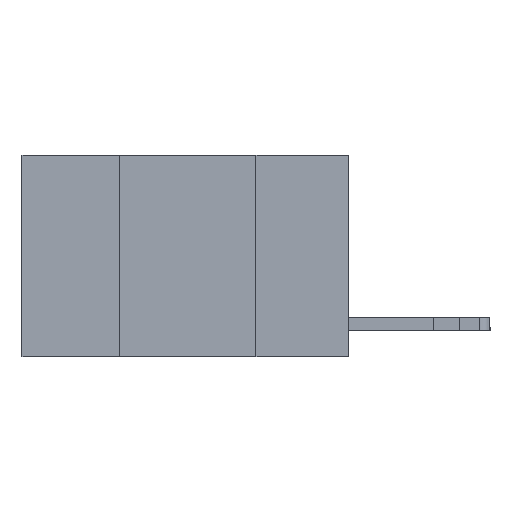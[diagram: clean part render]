
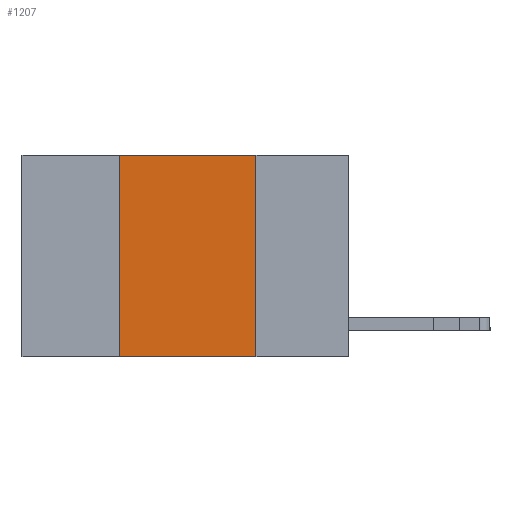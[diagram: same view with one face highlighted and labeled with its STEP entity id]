
A CAD part, left-side view. The second image highlights one B-rep face of the part: STEP entity #1207.
In plain terms, the highlighted planar face has unit normal (-1, 0, 0).
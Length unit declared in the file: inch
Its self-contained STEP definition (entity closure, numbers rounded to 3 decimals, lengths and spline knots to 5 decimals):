
#276 = ORIENTED_EDGE ( 'NONE', *, *, #12106, .F. ) ;
#777 = CARTESIAN_POINT ( 'NONE',  ( 0., 0.17, 0. ) ) ;
#1207 = ADVANCED_FACE ( 'NONE', ( #3936 ), #2541, .F. ) ;
#1278 = AXIS2_PLACEMENT_3D ( 'NONE', #9747, #12236, #2841 ) ;
#1428 = CARTESIAN_POINT ( 'NONE',  ( 0., 0.17, 0. ) ) ;
#1721 = EDGE_CURVE ( 'NONE', #3580, #10827, #12218, .T. ) ;
#2047 = VECTOR ( 'NONE', #6251, 39.37008 ) ;
#2541 = PLANE ( 'NONE',  #1278 ) ;
#2613 = LINE ( 'NONE', #4867, #14924 ) ;
#2841 = DIRECTION ( 'NONE',  ( 0., 0., -1. ) ) ;
#2943 = ORIENTED_EDGE ( 'NONE', *, *, #12474, .F. ) ;
#3580 = VERTEX_POINT ( 'NONE', #777 ) ;
#3683 = CARTESIAN_POINT ( 'NONE',  ( 0., 0.42, 0. ) ) ;
#3936 = FACE_OUTER_BOUND ( 'NONE', #4725, .T. ) ;
#4151 = EDGE_CURVE ( 'NONE', #6544, #10827, #9277, .T. ) ;
#4219 = CARTESIAN_POINT ( 'NONE',  ( 0., 0.42, 0. ) ) ;
#4725 = EDGE_LOOP ( 'NONE', ( #8576, #276, #2943, #12707 ) ) ;
#4867 = CARTESIAN_POINT ( 'NONE',  ( 0., 0.6, 0. ) ) ;
#6015 = LINE ( 'NONE', #3683, #11190 ) ;
#6251 = DIRECTION ( 'NONE',  ( 0., 0., -1. ) ) ;
#6544 = VERTEX_POINT ( 'NONE', #11555 ) ;
#6829 = DIRECTION ( 'NONE',  ( 0., -1., 0. ) ) ;
#6898 = VECTOR ( 'NONE', #6829, 39.37008 ) ;
#8013 = CARTESIAN_POINT ( 'NONE',  ( 0., 0.6, -0.37 ) ) ;
#8576 = ORIENTED_EDGE ( 'NONE', *, *, #1721, .F. ) ;
#8836 = CARTESIAN_POINT ( 'NONE',  ( 0., 0.17, -0.37 ) ) ;
#9277 = LINE ( 'NONE', #8013, #6898 ) ;
#9613 = VERTEX_POINT ( 'NONE', #4219 ) ;
#9747 = CARTESIAN_POINT ( 'NONE',  ( 0., 0.6, 0. ) ) ;
#10827 = VERTEX_POINT ( 'NONE', #8836 ) ;
#11190 = VECTOR ( 'NONE', #12212, 39.37008 ) ;
#11555 = CARTESIAN_POINT ( 'NONE',  ( 0., 0.42, -0.37 ) ) ;
#12074 = DIRECTION ( 'NONE',  ( 0., -1., 0. ) ) ;
#12106 = EDGE_CURVE ( 'NONE', #9613, #3580, #2613, .T. ) ;
#12212 = DIRECTION ( 'NONE',  ( 0., 0., 1. ) ) ;
#12218 = LINE ( 'NONE', #1428, #2047 ) ;
#12236 = DIRECTION ( 'NONE',  ( 1., 0., 0. ) ) ;
#12474 = EDGE_CURVE ( 'NONE', #6544, #9613, #6015, .T. ) ;
#12707 = ORIENTED_EDGE ( 'NONE', *, *, #4151, .T. ) ;
#14924 = VECTOR ( 'NONE', #12074, 39.37008 ) ;
